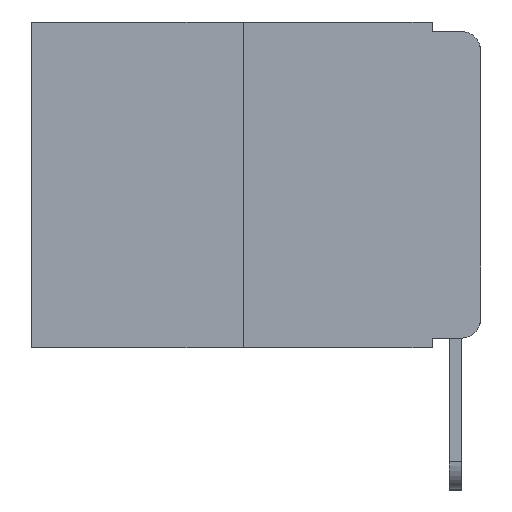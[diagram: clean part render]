
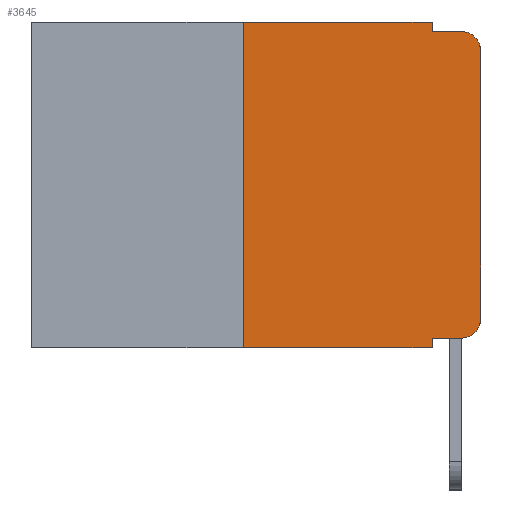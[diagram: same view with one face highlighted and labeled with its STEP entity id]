
A CAD part, left-side view. The second image highlights one B-rep face of the part: STEP entity #3645.
In plain terms, the highlighted planar face has unit normal (-1, 0, 0).
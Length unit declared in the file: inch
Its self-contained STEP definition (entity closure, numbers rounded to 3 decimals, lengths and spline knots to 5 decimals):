
#194 = ORIENTED_EDGE ( 'NONE', *, *, #8134, .F. ) ;
#387 = CARTESIAN_POINT ( 'NONE',  ( 0., 0.02, -0.333 ) ) ;
#649 = CARTESIAN_POINT ( 'NONE',  ( 0., 0., -0.03 ) ) ;
#652 = CARTESIAN_POINT ( 'NONE',  ( 0., 0.25, 0. ) ) ;
#824 = FACE_OUTER_BOUND ( 'NONE', #7198, .T. ) ;
#898 = DIRECTION ( 'NONE',  ( 1., 0., 0. ) ) ;
#933 = VERTEX_POINT ( 'NONE', #1420 ) ;
#1128 = LINE ( 'NONE', #9531, #2502 ) ;
#1420 = CARTESIAN_POINT ( 'NONE',  ( 0., 0.25, 0. ) ) ;
#1722 = AXIS2_PLACEMENT_3D ( 'NONE', #7845, #3021, #7771 ) ;
#1968 = VECTOR ( 'NONE', #15314, 39.37008 ) ;
#2018 = LINE ( 'NONE', #3141, #3914 ) ;
#2157 = CARTESIAN_POINT ( 'NONE',  ( 0., 0.051, -0.333 ) ) ;
#2283 = CARTESIAN_POINT ( 'NONE',  ( 0., 0.051, -0.343 ) ) ;
#2295 = CARTESIAN_POINT ( 'NONE',  ( 0., 0.051, 0. ) ) ;
#2381 = CARTESIAN_POINT ( 'NONE',  ( 0., 0.051, 0. ) ) ;
#2473 = LINE ( 'NONE', #9686, #12840 ) ;
#2502 = VECTOR ( 'NONE', #15338, 39.37008 ) ;
#2635 = EDGE_CURVE ( 'NONE', #14416, #10059, #11962, .T. ) ;
#2797 = VERTEX_POINT ( 'NONE', #2381 ) ;
#3021 = DIRECTION ( 'NONE',  ( -1., 0., 0. ) ) ;
#3127 = LINE ( 'NONE', #652, #10559 ) ;
#3141 = CARTESIAN_POINT ( 'NONE',  ( 0., 0.473, 0. ) ) ;
#3194 = DIRECTION ( 'NONE',  ( 0., 0., 1. ) ) ;
#3213 = DIRECTION ( 'NONE',  ( 0., 0., -1. ) ) ;
#3645 = ADVANCED_FACE ( 'NONE', ( #824 ), #10492, .F. ) ;
#3914 = VECTOR ( 'NONE', #5602, 39.37008 ) ;
#4363 = CARTESIAN_POINT ( 'NONE',  ( 0., 0., 0. ) ) ;
#4410 = EDGE_CURVE ( 'NONE', #12552, #15312, #11095, .T. ) ;
#4529 = EDGE_CURVE ( 'NONE', #10059, #12552, #5720, .T. ) ;
#4717 = CARTESIAN_POINT ( 'NONE',  ( 0., 0.473, 0. ) ) ;
#5255 = EDGE_CURVE ( 'NONE', #9262, #933, #3127, .T. ) ;
#5460 = EDGE_CURVE ( 'NONE', #9262, #6473, #1128, .T. ) ;
#5502 = CARTESIAN_POINT ( 'NONE',  ( 0., 0.02, -0.313 ) ) ;
#5602 = DIRECTION ( 'NONE',  ( 0., -1., 0. ) ) ;
#5720 = LINE ( 'NONE', #4363, #13890 ) ;
#5726 = ORIENTED_EDGE ( 'NONE', *, *, #12599, .F. ) ;
#5897 = ORIENTED_EDGE ( 'NONE', *, *, #2635, .T. ) ;
#5940 = ORIENTED_EDGE ( 'NONE', *, *, #4529, .T. ) ;
#6234 = VERTEX_POINT ( 'NONE', #10363 ) ;
#6473 = VERTEX_POINT ( 'NONE', #2283 ) ;
#7102 = CARTESIAN_POINT ( 'NONE',  ( 0., 0.02, -0.01 ) ) ;
#7198 = EDGE_LOOP ( 'NONE', ( #5940, #11423, #194, #5726, #9192, #14848, #12151, #13990, #9020, #5897 ) ) ;
#7771 = DIRECTION ( 'NONE',  ( 0., 0., -1. ) ) ;
#7845 = CARTESIAN_POINT ( 'NONE',  ( 0., 0.02, -0.03 ) ) ;
#7920 = CARTESIAN_POINT ( 'NONE',  ( 0., 0.051, -0.01 ) ) ;
#7929 = DIRECTION ( 'NONE',  ( 0., 0., 1. ) ) ;
#7950 = LINE ( 'NONE', #11752, #8580 ) ;
#8134 = EDGE_CURVE ( 'NONE', #6234, #15312, #15009, .T. ) ;
#8580 = VECTOR ( 'NONE', #11665, 39.37008 ) ;
#9020 = ORIENTED_EDGE ( 'NONE', *, *, #13816, .T. ) ;
#9192 = ORIENTED_EDGE ( 'NONE', *, *, #12046, .F. ) ;
#9262 = VERTEX_POINT ( 'NONE', #14620 ) ;
#9415 = LINE ( 'NONE', #2295, #11580 ) ;
#9424 = AXIS2_PLACEMENT_3D ( 'NONE', #5502, #11514, #15105 ) ;
#9531 = CARTESIAN_POINT ( 'NONE',  ( 0., 0.473, -0.343 ) ) ;
#9686 = CARTESIAN_POINT ( 'NONE',  ( 0., 0.051, 0. ) ) ;
#9876 = CARTESIAN_POINT ( 'NONE',  ( 0., 0., -0.313 ) ) ;
#10059 = VERTEX_POINT ( 'NONE', #9876 ) ;
#10363 = CARTESIAN_POINT ( 'NONE',  ( 0., 0.051, -0.01 ) ) ;
#10492 = PLANE ( 'NONE',  #14506 ) ;
#10559 = VECTOR ( 'NONE', #3194, 39.37008 ) ;
#11095 = CIRCLE ( 'NONE', #1722, 0.02 ) ;
#11423 = ORIENTED_EDGE ( 'NONE', *, *, #4410, .T. ) ;
#11502 = VERTEX_POINT ( 'NONE', #2157 ) ;
#11514 = DIRECTION ( 'NONE',  ( -1., 0., 0. ) ) ;
#11580 = VECTOR ( 'NONE', #15475, 39.37008 ) ;
#11665 = DIRECTION ( 'NONE',  ( 0., -1., 0. ) ) ;
#11752 = CARTESIAN_POINT ( 'NONE',  ( 0., 0.051, -0.333 ) ) ;
#11962 = CIRCLE ( 'NONE', #9424, 0.02 ) ;
#12046 = EDGE_CURVE ( 'NONE', #933, #2797, #2018, .T. ) ;
#12151 = ORIENTED_EDGE ( 'NONE', *, *, #5460, .T. ) ;
#12552 = VERTEX_POINT ( 'NONE', #649 ) ;
#12599 = EDGE_CURVE ( 'NONE', #2797, #6234, #2473, .T. ) ;
#12840 = VECTOR ( 'NONE', #13100, 39.37008 ) ;
#13096 = EDGE_CURVE ( 'NONE', #11502, #6473, #9415, .T. ) ;
#13100 = DIRECTION ( 'NONE',  ( 0., 0., -1. ) ) ;
#13816 = EDGE_CURVE ( 'NONE', #11502, #14416, #7950, .T. ) ;
#13890 = VECTOR ( 'NONE', #7929, 39.37008 ) ;
#13990 = ORIENTED_EDGE ( 'NONE', *, *, #13096, .F. ) ;
#14416 = VERTEX_POINT ( 'NONE', #387 ) ;
#14506 = AXIS2_PLACEMENT_3D ( 'NONE', #4717, #898, #3213 ) ;
#14620 = CARTESIAN_POINT ( 'NONE',  ( 0., 0.25, -0.343 ) ) ;
#14848 = ORIENTED_EDGE ( 'NONE', *, *, #5255, .F. ) ;
#15009 = LINE ( 'NONE', #7920, #1968 ) ;
#15105 = DIRECTION ( 'NONE',  ( 0., 0., -1. ) ) ;
#15312 = VERTEX_POINT ( 'NONE', #7102 ) ;
#15314 = DIRECTION ( 'NONE',  ( 0., -1., 0. ) ) ;
#15338 = DIRECTION ( 'NONE',  ( 0., -1., 0. ) ) ;
#15475 = DIRECTION ( 'NONE',  ( 0., 0., -1. ) ) ;
